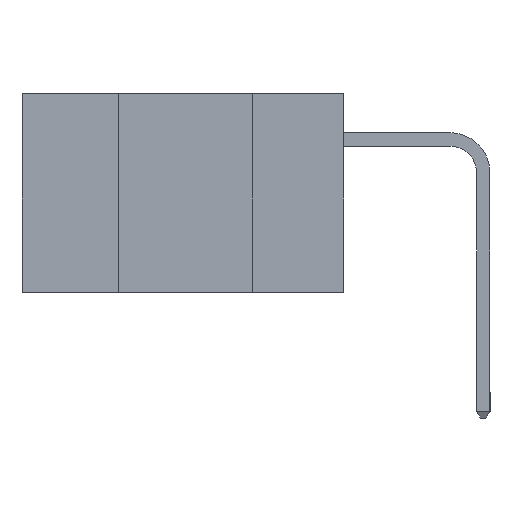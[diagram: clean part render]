
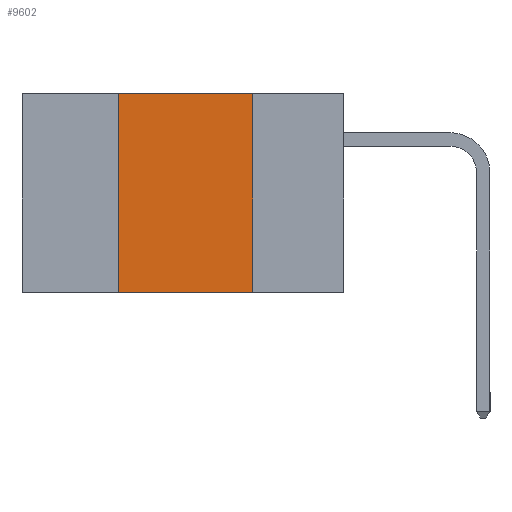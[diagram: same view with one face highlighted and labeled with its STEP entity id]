
A CAD part, left-side view. The second image highlights one B-rep face of the part: STEP entity #9602.
In plain terms, the highlighted planar face has unit normal (-1, 0, 0).
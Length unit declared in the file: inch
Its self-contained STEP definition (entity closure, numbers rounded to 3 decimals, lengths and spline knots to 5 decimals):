
#737 = VECTOR ( 'NONE', #4181, 39.37008 ) ;
#963 = LINE ( 'NONE', #3655, #3171 ) ;
#1177 = EDGE_CURVE ( 'NONE', #7028, #8733, #5962, .T. ) ;
#1325 = AXIS2_PLACEMENT_3D ( 'NONE', #3264, #9716, #4911 ) ;
#1933 = VECTOR ( 'NONE', #7388, 39.37008 ) ;
#2070 = CARTESIAN_POINT ( 'NONE',  ( 0., 0.17, 0. ) ) ;
#2493 = EDGE_LOOP ( 'NONE', ( #3680, #2773, #8746, #6102 ) ) ;
#2600 = EDGE_CURVE ( 'NONE', #8733, #2697, #963, .T. ) ;
#2697 = VERTEX_POINT ( 'NONE', #2070 ) ;
#2773 = ORIENTED_EDGE ( 'NONE', *, *, #2600, .F. ) ;
#3171 = VECTOR ( 'NONE', #8801, 39.37008 ) ;
#3264 = CARTESIAN_POINT ( 'NONE',  ( 0., 0.6, 0. ) ) ;
#3348 = CARTESIAN_POINT ( 'NONE',  ( 0., 0.6, -0.37 ) ) ;
#3655 = CARTESIAN_POINT ( 'NONE',  ( 0., 0.6, 0. ) ) ;
#3680 = ORIENTED_EDGE ( 'NONE', *, *, #7107, .F. ) ;
#3814 = VECTOR ( 'NONE', #4732, 39.37008 ) ;
#4181 = DIRECTION ( 'NONE',  ( 0., -1., 0. ) ) ;
#4631 = CARTESIAN_POINT ( 'NONE',  ( 0., 0.42, 0. ) ) ;
#4732 = DIRECTION ( 'NONE',  ( 0., 0., 1. ) ) ;
#4911 = DIRECTION ( 'NONE',  ( 0., 0., -1. ) ) ;
#5071 = VERTEX_POINT ( 'NONE', #7749 ) ;
#5134 = LINE ( 'NONE', #3348, #737 ) ;
#5962 = LINE ( 'NONE', #4631, #3814 ) ;
#6102 = ORIENTED_EDGE ( 'NONE', *, *, #9022, .T. ) ;
#7028 = VERTEX_POINT ( 'NONE', #7170 ) ;
#7107 = EDGE_CURVE ( 'NONE', #2697, #5071, #10291, .T. ) ;
#7170 = CARTESIAN_POINT ( 'NONE',  ( 0., 0.42, -0.37 ) ) ;
#7388 = DIRECTION ( 'NONE',  ( 0., 0., -1. ) ) ;
#7426 = CARTESIAN_POINT ( 'NONE',  ( 0., 0.17, 0. ) ) ;
#7749 = CARTESIAN_POINT ( 'NONE',  ( 0., 0.17, -0.37 ) ) ;
#8733 = VERTEX_POINT ( 'NONE', #10222 ) ;
#8746 = ORIENTED_EDGE ( 'NONE', *, *, #1177, .F. ) ;
#8801 = DIRECTION ( 'NONE',  ( 0., -1., 0. ) ) ;
#8925 = PLANE ( 'NONE',  #1325 ) ;
#9022 = EDGE_CURVE ( 'NONE', #7028, #5071, #5134, .T. ) ;
#9602 = ADVANCED_FACE ( 'NONE', ( #9768 ), #8925, .F. ) ;
#9716 = DIRECTION ( 'NONE',  ( 1., 0., 0. ) ) ;
#9768 = FACE_OUTER_BOUND ( 'NONE', #2493, .T. ) ;
#10222 = CARTESIAN_POINT ( 'NONE',  ( 0., 0.42, 0. ) ) ;
#10291 = LINE ( 'NONE', #7426, #1933 ) ;
